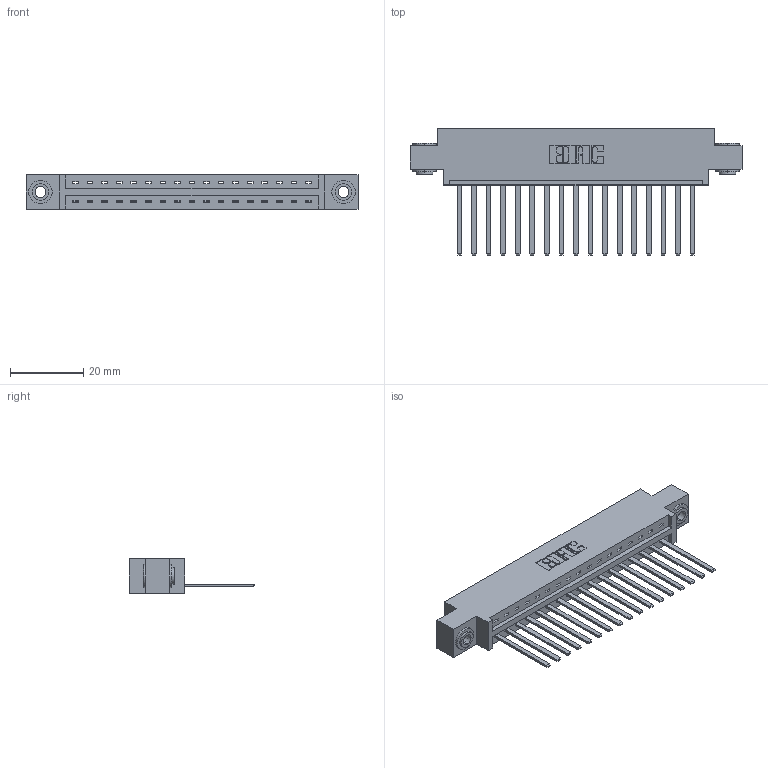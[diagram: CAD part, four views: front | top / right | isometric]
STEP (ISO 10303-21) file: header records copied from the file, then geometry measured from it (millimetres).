
FILE_DESCRIPTION (( 'STEP AP203' ), '1' );
FILE_NAME ('337-017-544-603.STEP', '2019-09-28T19:15:22', ( '' ), ( '' ), 'SwSTEP 2.0', 'SolidWorks 2016', '' );
FILE_SCHEMA (( 'CONFIG_CONTROL_DESIGN' ));
Length unit declared in the file: inch
Products named in the file (4): 345-250-002_345-250-002-102; 337-017-544-603; 337 Part_0.170 Offset - 0.156 Dia-TH; 345-292-001_345-293-144
Assembly tree (20 placements, depth 2):
  337-017-544-603
    337 Part_0.170 Offset - 0.156 Dia-TH
    345-292-001_345-293-144  x17
    345-250-002_345-250-002-102  x2
Bounding box: 90.37 x 34.3 x 9.4 mm (x, y, z)
Volume: 9178.7 mm3; surface area: 10322.9 mm2
Topology: 20 solids, 20 shells, 1108 faces, 3289 edges, 2166 vertices
Faces by surface type: plane 798, cylinder 302, cone 8
Entity records: 16468 total; most frequent: CARTESIAN_POINT 2844, ORIENTED_EDGE 2790, DIRECTION 2475, EDGE_CURVE 1395, LINE 1247, VECTOR 1247, VERTEX_POINT 926, AXIS2_PLACEMENT_3D 614
